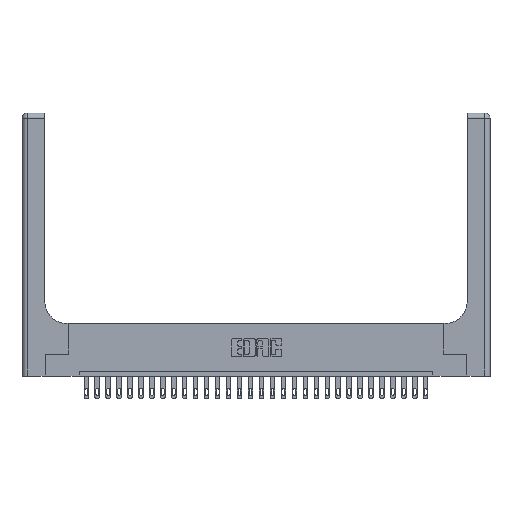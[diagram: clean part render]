
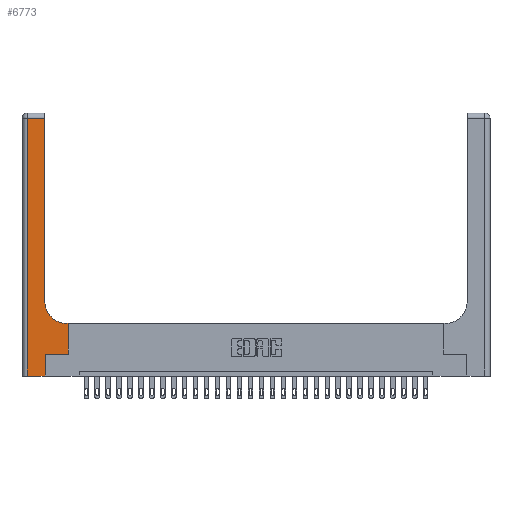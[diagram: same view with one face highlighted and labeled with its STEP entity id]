
A CAD part, top view. The second image highlights one B-rep face of the part: STEP entity #6773.
In plain terms, the highlighted planar face has unit normal (0, 0, 1).
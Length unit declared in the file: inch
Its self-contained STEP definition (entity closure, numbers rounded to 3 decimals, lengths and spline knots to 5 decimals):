
#67 = DIRECTION ( 'NONE',  ( 1., 0., 0. ) ) ;
#166 = CARTESIAN_POINT ( 'NONE',  ( 0.265, 0., 0.37 ) ) ;
#450 = EDGE_CURVE ( 'NONE', #24778, #25175, #14962, .T. ) ;
#1055 = EDGE_CURVE ( 'NONE', #13298, #10614, #13827, .T. ) ;
#1966 = CARTESIAN_POINT ( 'NONE',  ( 0.51, 0.85, 0.37 ) ) ;
#1976 = CARTESIAN_POINT ( 'NONE',  ( 0.265, 0.25, 0.37 ) ) ;
#3197 = CARTESIAN_POINT ( 'NONE',  ( 0.528, 0.25, 0.37 ) ) ;
#3377 = VERTEX_POINT ( 'NONE', #7249 ) ;
#4241 = DIRECTION ( 'NONE',  ( 0., 1., 0. ) ) ;
#4418 = DIRECTION ( 'NONE',  ( 0., -1., 0. ) ) ;
#4446 = ORIENTED_EDGE ( 'NONE', *, *, #10595, .T. ) ;
#4788 = EDGE_CURVE ( 'NONE', #17108, #24778, #16699, .T. ) ;
#6274 = CARTESIAN_POINT ( 'NONE',  ( 0.528, 0.6, 0.37 ) ) ;
#6481 = CARTESIAN_POINT ( 'NONE',  ( 0.06, 0., 0.37 ) ) ;
#6773 = ADVANCED_FACE ( 'NONE', ( #14592 ), #24768, .F. ) ;
#6903 = CARTESIAN_POINT ( 'NONE',  ( 0.528, 0.25, 0.37 ) ) ;
#7249 = CARTESIAN_POINT ( 'NONE',  ( 0.51, 0.6, 0.37 ) ) ;
#7489 = CARTESIAN_POINT ( 'NONE',  ( 0.26, 0.6, 0.37 ) ) ;
#7585 = ORIENTED_EDGE ( 'NONE', *, *, #1055, .T. ) ;
#8159 = CARTESIAN_POINT ( 'NONE',  ( 0.26, 3., 0.37 ) ) ;
#8702 = VERTEX_POINT ( 'NONE', #13019 ) ;
#8805 = AXIS2_PLACEMENT_3D ( 'NONE', #16362, #22609, #12718 ) ;
#9242 = ORIENTED_EDGE ( 'NONE', *, *, #19530, .T. ) ;
#9940 = DIRECTION ( 'NONE',  ( 0., 0., -1. ) ) ;
#10016 = CARTESIAN_POINT ( 'NONE',  ( 0.26, 2.94, 0.37 ) ) ;
#10595 = EDGE_CURVE ( 'NONE', #10614, #17108, #12307, .T. ) ;
#10614 = VERTEX_POINT ( 'NONE', #10016 ) ;
#10626 = LINE ( 'NONE', #1976, #26502 ) ;
#11983 = EDGE_CURVE ( 'NONE', #25175, #8702, #14617, .T. ) ;
#12307 = LINE ( 'NONE', #14179, #23140 ) ;
#12548 = ORIENTED_EDGE ( 'NONE', *, *, #450, .T. ) ;
#12718 = DIRECTION ( 'NONE',  ( -1., 0., 0. ) ) ;
#13019 = CARTESIAN_POINT ( 'NONE',  ( 0.265, 0.25, 0.37 ) ) ;
#13298 = VERTEX_POINT ( 'NONE', #24572 ) ;
#13692 = DIRECTION ( 'NONE',  ( -1., 0., 0. ) ) ;
#13827 = LINE ( 'NONE', #8159, #26295 ) ;
#14179 = CARTESIAN_POINT ( 'NONE',  ( 0., 2.94, 0.37 ) ) ;
#14592 = FACE_OUTER_BOUND ( 'NONE', #22726, .T. ) ;
#14617 = LINE ( 'NONE', #166, #19733 ) ;
#14962 = LINE ( 'NONE', #23238, #15525 ) ;
#15107 = ORIENTED_EDGE ( 'NONE', *, *, #4788, .T. ) ;
#15453 = ORIENTED_EDGE ( 'NONE', *, *, #16865, .T. ) ;
#15525 = VECTOR ( 'NONE', #17134, 39.37008 ) ;
#16057 = VERTEX_POINT ( 'NONE', #6274 ) ;
#16362 = CARTESIAN_POINT ( 'NONE',  ( 0., 3., 0.37 ) ) ;
#16406 = DIRECTION ( 'NONE',  ( 0., 1., 0. ) ) ;
#16699 = LINE ( 'NONE', #22929, #25566 ) ;
#16865 = EDGE_CURVE ( 'NONE', #3377, #13298, #22501, .T. ) ;
#17108 = VERTEX_POINT ( 'NONE', #25896 ) ;
#17134 = DIRECTION ( 'NONE',  ( 1., 0., 0. ) ) ;
#18979 = CARTESIAN_POINT ( 'NONE',  ( 0.265, 0., 0.37 ) ) ;
#19530 = EDGE_CURVE ( 'NONE', #16057, #3377, #22093, .T. ) ;
#19733 = VECTOR ( 'NONE', #4241, 39.37008 ) ;
#20387 = VERTEX_POINT ( 'NONE', #3197 ) ;
#21260 = DIRECTION ( 'NONE',  ( 0., 1., 0. ) ) ;
#21739 = EDGE_CURVE ( 'NONE', #8702, #20387, #10626, .T. ) ;
#21805 = VECTOR ( 'NONE', #21260, 39.37008 ) ;
#22093 = LINE ( 'NONE', #7489, #26003 ) ;
#22501 = CIRCLE ( 'NONE', #23368, 0.25 ) ;
#22609 = DIRECTION ( 'NONE',  ( 0., 0., -1. ) ) ;
#22726 = EDGE_LOOP ( 'NONE', ( #7585, #4446, #15107, #12548, #26210, #25680, #25157, #9242, #15453 ) ) ;
#22929 = CARTESIAN_POINT ( 'NONE',  ( 0.06, 3., 0.37 ) ) ;
#23140 = VECTOR ( 'NONE', #26654, 39.37008 ) ;
#23238 = CARTESIAN_POINT ( 'NONE',  ( 0., 0., 0.37 ) ) ;
#23368 = AXIS2_PLACEMENT_3D ( 'NONE', #1966, #9940, #24421 ) ;
#23681 = LINE ( 'NONE', #6903, #21805 ) ;
#24421 = DIRECTION ( 'NONE',  ( 1., 0., 0. ) ) ;
#24497 = EDGE_CURVE ( 'NONE', #20387, #16057, #23681, .T. ) ;
#24572 = CARTESIAN_POINT ( 'NONE',  ( 0.26, 0.85, 0.37 ) ) ;
#24768 = PLANE ( 'NONE',  #8805 ) ;
#24778 = VERTEX_POINT ( 'NONE', #6481 ) ;
#25157 = ORIENTED_EDGE ( 'NONE', *, *, #24497, .T. ) ;
#25175 = VERTEX_POINT ( 'NONE', #18979 ) ;
#25566 = VECTOR ( 'NONE', #4418, 39.37008 ) ;
#25680 = ORIENTED_EDGE ( 'NONE', *, *, #21739, .T. ) ;
#25896 = CARTESIAN_POINT ( 'NONE',  ( 0.06, 2.94, 0.37 ) ) ;
#26003 = VECTOR ( 'NONE', #13692, 39.37008 ) ;
#26210 = ORIENTED_EDGE ( 'NONE', *, *, #11983, .T. ) ;
#26295 = VECTOR ( 'NONE', #16406, 39.37008 ) ;
#26502 = VECTOR ( 'NONE', #67, 39.37008 ) ;
#26654 = DIRECTION ( 'NONE',  ( -1., 0., 0. ) ) ;
